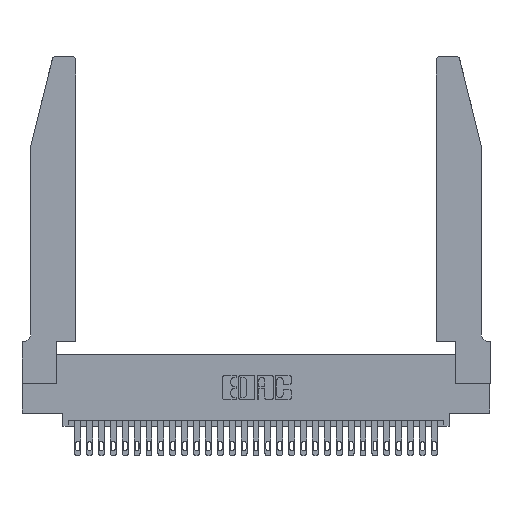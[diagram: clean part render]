
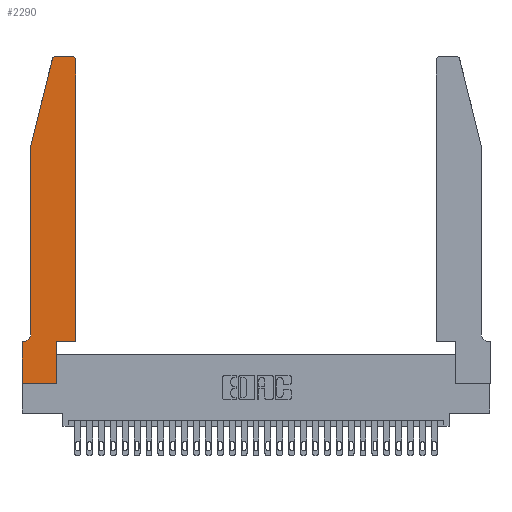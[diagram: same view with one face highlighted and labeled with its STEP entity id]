
A CAD part, top view. The second image highlights one B-rep face of the part: STEP entity #2290.
In plain terms, the highlighted planar face has unit normal (0, 0, 1).
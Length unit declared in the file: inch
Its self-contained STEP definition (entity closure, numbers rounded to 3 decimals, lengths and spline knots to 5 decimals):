
#787 = ORIENTED_EDGE ( 'NONE', *, *, #14289, .T. ) ;
#862 = DIRECTION ( 'NONE',  ( 1., 0., 0. ) ) ;
#1039 = CARTESIAN_POINT ( 'NONE',  ( 0.0755, 2., 0.37 ) ) ;
#1138 = CARTESIAN_POINT ( 'NONE',  ( 0.2605, 2.75, 0.37 ) ) ;
#2241 = VERTEX_POINT ( 'NONE', #6708 ) ;
#2290 = ADVANCED_FACE ( 'NONE', ( #25086 ), #8681, .T. ) ;
#2589 = ORIENTED_EDGE ( 'NONE', *, *, #27488, .T. ) ;
#3543 = ORIENTED_EDGE ( 'NONE', *, *, #25261, .T. ) ;
#3821 = CARTESIAN_POINT ( 'NONE',  ( 0., 0.35, 0.37 ) ) ;
#3844 = VECTOR ( 'NONE', #20604, 39.37008 ) ;
#4313 = EDGE_CURVE ( 'NONE', #26274, #12651, #22089, .T. ) ;
#4473 = VECTOR ( 'NONE', #18067, 39.37008 ) ;
#4630 = VECTOR ( 'NONE', #26834, 39.37008 ) ;
#5207 = CARTESIAN_POINT ( 'NONE',  ( 0.2865, 0., 0.37 ) ) ;
#5254 = LINE ( 'NONE', #12236, #18660 ) ;
#5662 = VECTOR ( 'NONE', #25779, 39.37008 ) ;
#6430 = EDGE_CURVE ( 'NONE', #25124, #24801, #13007, .T. ) ;
#6477 = DIRECTION ( 'NONE',  ( 0., 0., 1. ) ) ;
#6638 = DIRECTION ( 'NONE',  ( 1., 0., 0. ) ) ;
#6708 = CARTESIAN_POINT ( 'NONE',  ( 0.284, 2.75, 0.37 ) ) ;
#7467 = CARTESIAN_POINT ( 'NONE',  ( 0.4205, 2.72, 0.37 ) ) ;
#7575 = DIRECTION ( 'NONE',  ( 1., 0., 0. ) ) ;
#8057 = LINE ( 'NONE', #12633, #24400 ) ;
#8337 = LINE ( 'NONE', #1039, #13906 ) ;
#8365 = AXIS2_PLACEMENT_3D ( 'NONE', #10957, #13009, #19978 ) ;
#8681 = PLANE ( 'NONE',  #11336 ) ;
#9220 = ORIENTED_EDGE ( 'NONE', *, *, #9529, .T. ) ;
#9423 = CARTESIAN_POINT ( 'NONE',  ( 0.2865, 0.35, 0.37 ) ) ;
#9529 = EDGE_CURVE ( 'NONE', #13353, #23027, #19901, .T. ) ;
#10171 = CARTESIAN_POINT ( 'NONE',  ( 0.4505, 0.35, 0.37 ) ) ;
#10357 = DIRECTION ( 'NONE',  ( 0., -1., 0. ) ) ;
#10753 = LINE ( 'NONE', #22966, #4473 ) ;
#10943 = ORIENTED_EDGE ( 'NONE', *, *, #29387, .T. ) ;
#10957 = CARTESIAN_POINT ( 'NONE',  ( 0.0055, 0.42, 0.37 ) ) ;
#11065 = VERTEX_POINT ( 'NONE', #13088 ) ;
#11274 = ORIENTED_EDGE ( 'NONE', *, *, #14321, .T. ) ;
#11336 = AXIS2_PLACEMENT_3D ( 'NONE', #3821, #6477, #22805 ) ;
#11382 = ORIENTED_EDGE ( 'NONE', *, *, #6430, .T. ) ;
#11538 = VERTEX_POINT ( 'NONE', #5207 ) ;
#11675 = LINE ( 'NONE', #1138, #4630 ) ;
#12236 = CARTESIAN_POINT ( 'NONE',  ( 0.0755, 0.35, 0.37 ) ) ;
#12633 = CARTESIAN_POINT ( 'NONE',  ( 0., 0., 0.37 ) ) ;
#12651 = VERTEX_POINT ( 'NONE', #26930 ) ;
#13007 = CIRCLE ( 'NONE', #25767, 0.03 ) ;
#13009 = DIRECTION ( 'NONE',  ( 0., 0., -1. ) ) ;
#13088 = CARTESIAN_POINT ( 'NONE',  ( 0.25487, 2.72718, 0.37 ) ) ;
#13353 = VERTEX_POINT ( 'NONE', #9423 ) ;
#13906 = VECTOR ( 'NONE', #10357, 39.37008 ) ;
#13916 = DIRECTION ( 'NONE',  ( 0., 0., 1. ) ) ;
#14289 = EDGE_CURVE ( 'NONE', #22607, #11538, #24602, .T. ) ;
#14321 = EDGE_CURVE ( 'NONE', #23027, #25124, #18280, .T. ) ;
#14717 = EDGE_CURVE ( 'NONE', #12651, #27224, #5254, .T. ) ;
#15596 = VERTEX_POINT ( 'NONE', #26296 ) ;
#15709 = CARTESIAN_POINT ( 'NONE',  ( 0., 0., 0.37 ) ) ;
#15806 = LINE ( 'NONE', #20631, #22884 ) ;
#16026 = CARTESIAN_POINT ( 'NONE',  ( 0.4205, 2.75, 0.37 ) ) ;
#16858 = CARTESIAN_POINT ( 'NONE',  ( 0.0755, 0.42, 0.37 ) ) ;
#17017 = DIRECTION ( 'NONE',  ( -1., 0., 0. ) ) ;
#18067 = DIRECTION ( 'NONE',  ( -0.239, -0.971, 0. ) ) ;
#18280 = LINE ( 'NONE', #22897, #5662 ) ;
#18344 = EDGE_CURVE ( 'NONE', #11538, #13353, #15806, .T. ) ;
#18660 = VECTOR ( 'NONE', #17017, 39.37008 ) ;
#19020 = EDGE_CURVE ( 'NONE', #24801, #2241, #11675, .T. ) ;
#19130 = EDGE_CURVE ( 'NONE', #15596, #26274, #8337, .T. ) ;
#19901 = LINE ( 'NONE', #10171, #20667 ) ;
#19978 = DIRECTION ( 'NONE',  ( -1., 0., 0. ) ) ;
#20604 = DIRECTION ( 'NONE',  ( 1., 0., 0. ) ) ;
#20631 = CARTESIAN_POINT ( 'NONE',  ( 0.2865, 0.35, 0.37 ) ) ;
#20667 = VECTOR ( 'NONE', #862, 39.37008 ) ;
#20680 = CARTESIAN_POINT ( 'NONE',  ( 0.284, 2.72, 0.37 ) ) ;
#20981 = CARTESIAN_POINT ( 'NONE',  ( 0., 0., 0.37 ) ) ;
#21789 = DIRECTION ( 'NONE',  ( 0., 0., 1. ) ) ;
#22089 = CIRCLE ( 'NONE', #8365, 0.07 ) ;
#22112 = CARTESIAN_POINT ( 'NONE',  ( 0.4505, 2.72, 0.37 ) ) ;
#22403 = DIRECTION ( 'NONE',  ( 0., -1., 0. ) ) ;
#22607 = VERTEX_POINT ( 'NONE', #20981 ) ;
#22805 = DIRECTION ( 'NONE',  ( 1., 0., 0. ) ) ;
#22884 = VECTOR ( 'NONE', #27765, 39.37008 ) ;
#22897 = CARTESIAN_POINT ( 'NONE',  ( 0.4505, 0.35, 0.37 ) ) ;
#22966 = CARTESIAN_POINT ( 'NONE',  ( 0.0755, 2., 0.37 ) ) ;
#23027 = VERTEX_POINT ( 'NONE', #27550 ) ;
#23483 = ORIENTED_EDGE ( 'NONE', *, *, #19020, .T. ) ;
#24191 = EDGE_LOOP ( 'NONE', ( #23483, #10943, #3543, #25233, #29593, #27580, #2589, #787, #26801, #9220, #11274, #11382 ) ) ;
#24400 = VECTOR ( 'NONE', #22403, 39.37008 ) ;
#24602 = LINE ( 'NONE', #15709, #3844 ) ;
#24801 = VERTEX_POINT ( 'NONE', #16026 ) ;
#25086 = FACE_OUTER_BOUND ( 'NONE', #24191, .T. ) ;
#25124 = VERTEX_POINT ( 'NONE', #22112 ) ;
#25233 = ORIENTED_EDGE ( 'NONE', *, *, #19130, .T. ) ;
#25261 = EDGE_CURVE ( 'NONE', #11065, #15596, #10753, .T. ) ;
#25418 = AXIS2_PLACEMENT_3D ( 'NONE', #20680, #13916, #6638 ) ;
#25767 = AXIS2_PLACEMENT_3D ( 'NONE', #7467, #21789, #7575 ) ;
#25779 = DIRECTION ( 'NONE',  ( 0., 1., 0. ) ) ;
#26274 = VERTEX_POINT ( 'NONE', #16858 ) ;
#26296 = CARTESIAN_POINT ( 'NONE',  ( 0.0755, 2., 0.37 ) ) ;
#26801 = ORIENTED_EDGE ( 'NONE', *, *, #18344, .T. ) ;
#26834 = DIRECTION ( 'NONE',  ( -1., 0., 0. ) ) ;
#26930 = CARTESIAN_POINT ( 'NONE',  ( 0.0055, 0.35, 0.37 ) ) ;
#27224 = VERTEX_POINT ( 'NONE', #30039 ) ;
#27488 = EDGE_CURVE ( 'NONE', #27224, #22607, #8057, .T. ) ;
#27550 = CARTESIAN_POINT ( 'NONE',  ( 0.4505, 0.35, 0.37 ) ) ;
#27580 = ORIENTED_EDGE ( 'NONE', *, *, #14717, .T. ) ;
#27765 = DIRECTION ( 'NONE',  ( 0., 1., 0. ) ) ;
#28355 = CIRCLE ( 'NONE', #25418, 0.03 ) ;
#29387 = EDGE_CURVE ( 'NONE', #2241, #11065, #28355, .T. ) ;
#29593 = ORIENTED_EDGE ( 'NONE', *, *, #4313, .T. ) ;
#30039 = CARTESIAN_POINT ( 'NONE',  ( 0., 0.35, 0.37 ) ) ;
